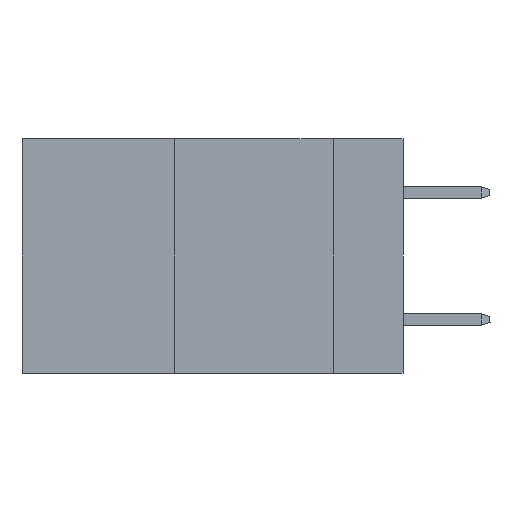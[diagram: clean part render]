
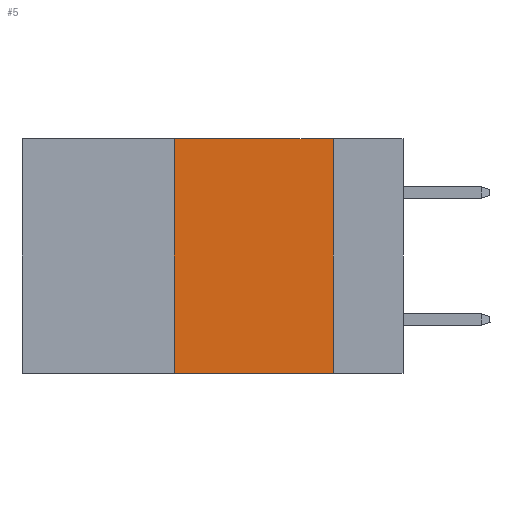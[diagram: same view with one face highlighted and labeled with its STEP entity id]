
A CAD part, left-side view. The second image highlights one B-rep face of the part: STEP entity #5.
In plain terms, the highlighted planar face has unit normal (-1, 0, 0).
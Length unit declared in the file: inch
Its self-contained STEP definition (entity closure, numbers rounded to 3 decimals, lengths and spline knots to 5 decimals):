
#5 = ADVANCED_FACE ( 'NONE', ( #5697 ), #16008, .F. ) ;
#879 = DIRECTION ( 'NONE',  ( 0., -1., 0. ) ) ;
#3292 = EDGE_CURVE ( 'NONE', #15306, #24215, #16269, .T. ) ;
#4130 = DIRECTION ( 'NONE',  ( 0., 0., -1. ) ) ;
#4297 = CARTESIAN_POINT ( 'NONE',  ( 0., 0.11, 0. ) ) ;
#4892 = EDGE_CURVE ( 'NONE', #15306, #7674, #21165, .T. ) ;
#5697 = FACE_OUTER_BOUND ( 'NONE', #9198, .T. ) ;
#6080 = CARTESIAN_POINT ( 'NONE',  ( 0., 0.6, 0. ) ) ;
#7155 = CARTESIAN_POINT ( 'NONE',  ( 0., 0.6, -0.37 ) ) ;
#7336 = ORIENTED_EDGE ( 'NONE', *, *, #3292, .F. ) ;
#7454 = CARTESIAN_POINT ( 'NONE',  ( 0., 0.36, 0. ) ) ;
#7674 = VERTEX_POINT ( 'NONE', #20528 ) ;
#8040 = ORIENTED_EDGE ( 'NONE', *, *, #21564, .F. ) ;
#9198 = EDGE_LOOP ( 'NONE', ( #8040, #12034, #7336, #22288 ) ) ;
#11196 = DIRECTION ( 'NONE',  ( 0., 0., -1. ) ) ;
#12034 = ORIENTED_EDGE ( 'NONE', *, *, #15043, .F. ) ;
#12532 = VECTOR ( 'NONE', #879, 39.37008 ) ;
#13518 = VERTEX_POINT ( 'NONE', #4297 ) ;
#14532 = VECTOR ( 'NONE', #11196, 39.37008 ) ;
#15043 = EDGE_CURVE ( 'NONE', #24215, #13518, #24907, .T. ) ;
#15306 = VERTEX_POINT ( 'NONE', #24222 ) ;
#16008 = PLANE ( 'NONE',  #21384 ) ;
#16269 = LINE ( 'NONE', #18639, #23415 ) ;
#16532 = DIRECTION ( 'NONE',  ( 0., 0., 1. ) ) ;
#18639 = CARTESIAN_POINT ( 'NONE',  ( 0., 0.36, 0. ) ) ;
#18817 = CARTESIAN_POINT ( 'NONE',  ( 0., 0.6, 0. ) ) ;
#20528 = CARTESIAN_POINT ( 'NONE',  ( 0., 0.11, -0.37 ) ) ;
#20927 = DIRECTION ( 'NONE',  ( 0., -1., 0. ) ) ;
#21165 = LINE ( 'NONE', #7155, #12532 ) ;
#21384 = AXIS2_PLACEMENT_3D ( 'NONE', #6080, #22074, #4130 ) ;
#21564 = EDGE_CURVE ( 'NONE', #13518, #7674, #23560, .T. ) ;
#21929 = VECTOR ( 'NONE', #20927, 39.37008 ) ;
#22074 = DIRECTION ( 'NONE',  ( 1., 0., 0. ) ) ;
#22288 = ORIENTED_EDGE ( 'NONE', *, *, #4892, .T. ) ;
#23415 = VECTOR ( 'NONE', #16532, 39.37008 ) ;
#23560 = LINE ( 'NONE', #25680, #14532 ) ;
#24215 = VERTEX_POINT ( 'NONE', #7454 ) ;
#24222 = CARTESIAN_POINT ( 'NONE',  ( 0., 0.36, -0.37 ) ) ;
#24907 = LINE ( 'NONE', #18817, #21929 ) ;
#25680 = CARTESIAN_POINT ( 'NONE',  ( 0., 0.11, 0. ) ) ;
